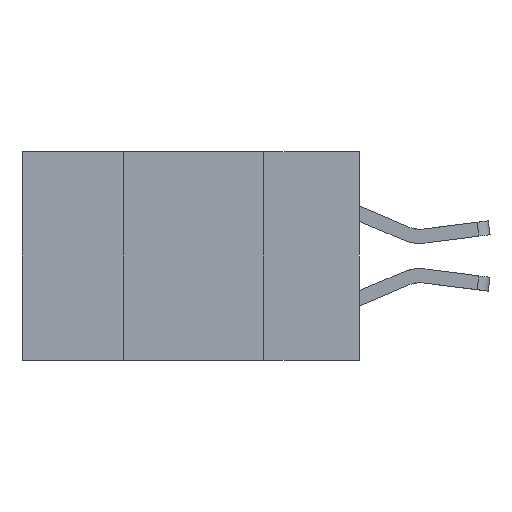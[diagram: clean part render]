
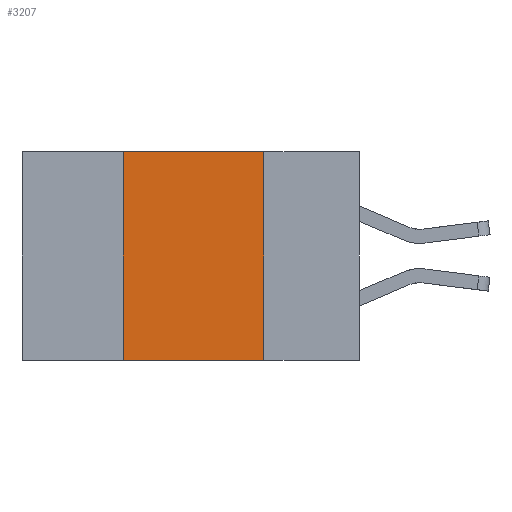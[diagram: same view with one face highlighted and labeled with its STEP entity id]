
A CAD part, left-side view. The second image highlights one B-rep face of the part: STEP entity #3207.
In plain terms, the highlighted planar face has unit normal (-1, 0, 0).
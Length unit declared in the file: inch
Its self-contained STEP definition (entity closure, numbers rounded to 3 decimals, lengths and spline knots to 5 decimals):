
#122 = EDGE_CURVE ( 'NONE', #1173, #5282, #2225, .T. ) ;
#429 = CARTESIAN_POINT ( 'NONE',  ( 0., 0.17, -0.37 ) ) ;
#994 = DIRECTION ( 'NONE',  ( 0., -1., 0. ) ) ;
#1173 = VERTEX_POINT ( 'NONE', #4231 ) ;
#1224 = VERTEX_POINT ( 'NONE', #429 ) ;
#1515 = CARTESIAN_POINT ( 'NONE',  ( 0., 0.6, 0. ) ) ;
#2225 = LINE ( 'NONE', #1515, #10649 ) ;
#2324 = VECTOR ( 'NONE', #3354, 39.37008 ) ;
#3041 = LINE ( 'NONE', #12370, #2324 ) ;
#3207 = ADVANCED_FACE ( 'NONE', ( #12604 ), #4975, .F. ) ;
#3213 = DIRECTION ( 'NONE',  ( 1., 0., 0. ) ) ;
#3309 = DIRECTION ( 'NONE',  ( 0., 0., -1. ) ) ;
#3354 = DIRECTION ( 'NONE',  ( 0., -1., 0. ) ) ;
#3443 = ORIENTED_EDGE ( 'NONE', *, *, #122, .F. ) ;
#4212 = CARTESIAN_POINT ( 'NONE',  ( 0., 0.17, 0. ) ) ;
#4217 = VERTEX_POINT ( 'NONE', #7058 ) ;
#4231 = CARTESIAN_POINT ( 'NONE',  ( 0., 0.42, 0. ) ) ;
#4521 = ORIENTED_EDGE ( 'NONE', *, *, #6004, .F. ) ;
#4975 = PLANE ( 'NONE',  #11752 ) ;
#5282 = VERTEX_POINT ( 'NONE', #9573 ) ;
#6004 = EDGE_CURVE ( 'NONE', #4217, #1173, #13748, .T. ) ;
#6339 = CARTESIAN_POINT ( 'NONE',  ( 0., 0.42, 0. ) ) ;
#6688 = DIRECTION ( 'NONE',  ( 0., 0., 1. ) ) ;
#7058 = CARTESIAN_POINT ( 'NONE',  ( 0., 0.42, -0.37 ) ) ;
#7214 = VECTOR ( 'NONE', #9742, 39.37008 ) ;
#7426 = EDGE_CURVE ( 'NONE', #4217, #1224, #3041, .T. ) ;
#7494 = ORIENTED_EDGE ( 'NONE', *, *, #7426, .T. ) ;
#7785 = EDGE_LOOP ( 'NONE', ( #13675, #3443, #4521, #7494 ) ) ;
#9573 = CARTESIAN_POINT ( 'NONE',  ( 0., 0.17, 0. ) ) ;
#9742 = DIRECTION ( 'NONE',  ( 0., 0., -1. ) ) ;
#10257 = CARTESIAN_POINT ( 'NONE',  ( 0., 0.6, 0. ) ) ;
#10564 = EDGE_CURVE ( 'NONE', #5282, #1224, #10700, .T. ) ;
#10649 = VECTOR ( 'NONE', #994, 39.37008 ) ;
#10700 = LINE ( 'NONE', #4212, #7214 ) ;
#11210 = VECTOR ( 'NONE', #6688, 39.37008 ) ;
#11752 = AXIS2_PLACEMENT_3D ( 'NONE', #10257, #3213, #3309 ) ;
#12370 = CARTESIAN_POINT ( 'NONE',  ( 0., 0.6, -0.37 ) ) ;
#12604 = FACE_OUTER_BOUND ( 'NONE', #7785, .T. ) ;
#13675 = ORIENTED_EDGE ( 'NONE', *, *, #10564, .F. ) ;
#13748 = LINE ( 'NONE', #6339, #11210 ) ;
